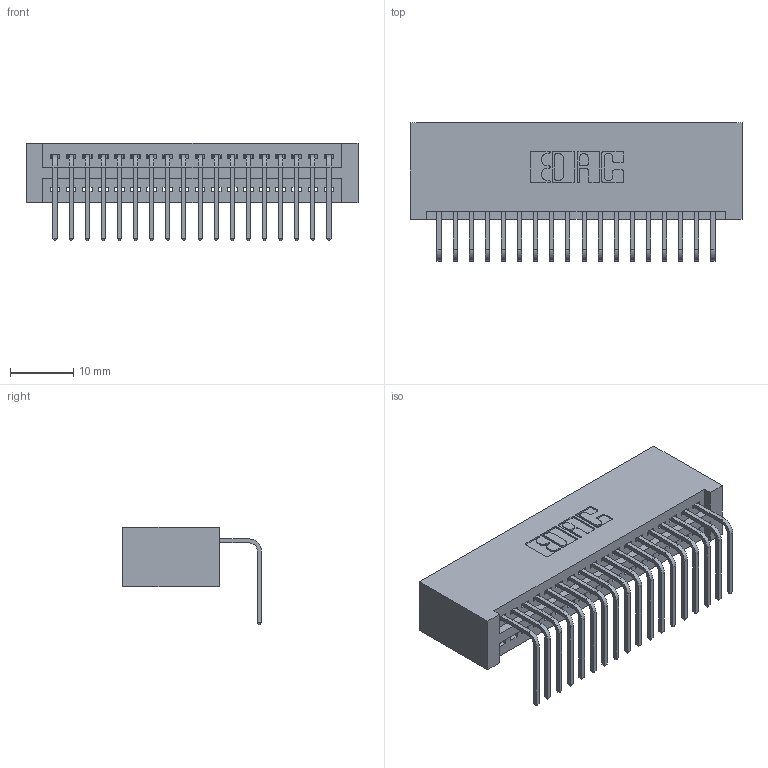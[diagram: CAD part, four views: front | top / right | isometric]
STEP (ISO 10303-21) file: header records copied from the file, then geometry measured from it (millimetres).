
FILE_DESCRIPTION (( 'STEP AP203' ), '1' );
FILE_NAME ('345-018-558-101.STEP', '2019-10-10T12:22:40', ( '' ), ( '' ), 'SwSTEP 2.0', 'SolidWorks 2016', '' );
FILE_SCHEMA (( 'CONFIG_CONTROL_DESIGN' ));
Length unit declared in the file: inch
Products named in the file (3): 345-292-001_558 Tail - 2; 345-018-558-101; 345 Part_No Mounting Lugs
Assembly tree (19 placements, depth 2):
  345-018-558-101
    345 Part_No Mounting Lugs
    345-292-001_558 Tail - 2  x18
Bounding box: 52.32 x 21.83 x 15.37 mm (x, y, z)
Volume: 5417.5 mm3; surface area: 7415.7 mm2
Topology: 19 solids, 19 shells, 1198 faces, 3593 edges, 2370 vertices
Faces by surface type: plane 832, cylinder 366
Entity records: 16585 total; most frequent: CARTESIAN_POINT 2882, ORIENTED_EDGE 2834, DIRECTION 2545, EDGE_CURVE 1417, LINE 1221, VECTOR 1221, VERTEX_POINT 942, AXIS2_PLACEMENT_3D 662
